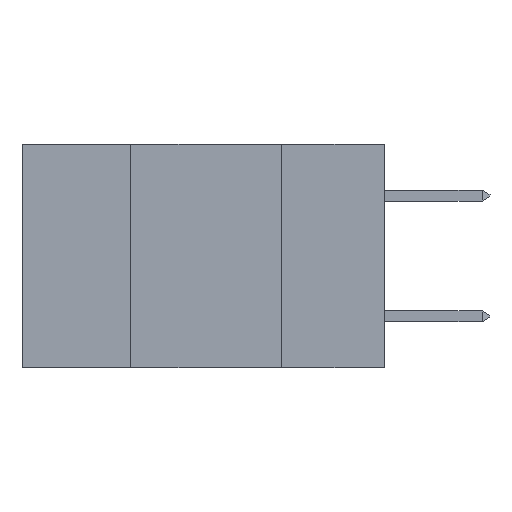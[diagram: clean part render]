
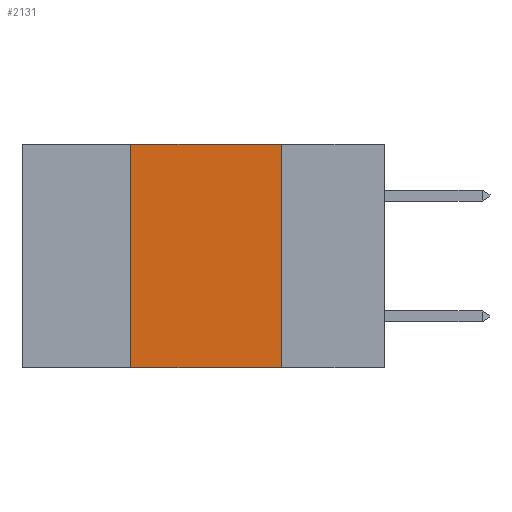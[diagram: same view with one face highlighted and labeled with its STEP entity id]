
A CAD part, left-side view. The second image highlights one B-rep face of the part: STEP entity #2131.
In plain terms, the highlighted planar face has unit normal (-1, 0, 0).
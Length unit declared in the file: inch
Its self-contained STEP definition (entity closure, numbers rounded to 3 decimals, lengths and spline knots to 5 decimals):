
#413 = CARTESIAN_POINT ( 'NONE',  ( 0., 0.42, 0. ) ) ;
#755 = LINE ( 'NONE', #12786, #13240 ) ;
#1171 = CARTESIAN_POINT ( 'NONE',  ( 0., 0.17, -0.37 ) ) ;
#1520 = VERTEX_POINT ( 'NONE', #1171 ) ;
#1821 = VERTEX_POINT ( 'NONE', #7901 ) ;
#2131 = ADVANCED_FACE ( 'NONE', ( #11432 ), #11680, .F. ) ;
#2383 = LINE ( 'NONE', #6045, #12382 ) ;
#2476 = VECTOR ( 'NONE', #11232, 39.37008 ) ;
#2914 = DIRECTION ( 'NONE',  ( 0., 0., 1. ) ) ;
#4854 = LINE ( 'NONE', #413, #14025 ) ;
#5162 = CARTESIAN_POINT ( 'NONE',  ( 0., 0.42, 0. ) ) ;
#6045 = CARTESIAN_POINT ( 'NONE',  ( 0., 0.6, 0. ) ) ;
#6496 = CARTESIAN_POINT ( 'NONE',  ( 0., 0.17, 0. ) ) ;
#6823 = DIRECTION ( 'NONE',  ( 0., -1., 0. ) ) ;
#6924 = DIRECTION ( 'NONE',  ( 1., 0., 0. ) ) ;
#6982 = EDGE_LOOP ( 'NONE', ( #10918, #13888, #10572, #9052 ) ) ;
#7901 = CARTESIAN_POINT ( 'NONE',  ( 0., 0.42, -0.37 ) ) ;
#8477 = EDGE_CURVE ( 'NONE', #1821, #15465, #4854, .T. ) ;
#9052 = ORIENTED_EDGE ( 'NONE', *, *, #14442, .T. ) ;
#10051 = CARTESIAN_POINT ( 'NONE',  ( 0., 0.17, 0. ) ) ;
#10572 = ORIENTED_EDGE ( 'NONE', *, *, #8477, .F. ) ;
#10918 = ORIENTED_EDGE ( 'NONE', *, *, #10987, .F. ) ;
#10987 = EDGE_CURVE ( 'NONE', #14907, #1520, #11728, .T. ) ;
#11232 = DIRECTION ( 'NONE',  ( 0., 0., -1. ) ) ;
#11296 = AXIS2_PLACEMENT_3D ( 'NONE', #12883, #6924, #15204 ) ;
#11432 = FACE_OUTER_BOUND ( 'NONE', #6982, .T. ) ;
#11442 = EDGE_CURVE ( 'NONE', #15465, #14907, #2383, .T. ) ;
#11680 = PLANE ( 'NONE',  #11296 ) ;
#11728 = LINE ( 'NONE', #10051, #2476 ) ;
#12382 = VECTOR ( 'NONE', #14380, 39.37008 ) ;
#12786 = CARTESIAN_POINT ( 'NONE',  ( 0., 0.6, -0.37 ) ) ;
#12883 = CARTESIAN_POINT ( 'NONE',  ( 0., 0.6, 0. ) ) ;
#13240 = VECTOR ( 'NONE', #6823, 39.37008 ) ;
#13888 = ORIENTED_EDGE ( 'NONE', *, *, #11442, .F. ) ;
#14025 = VECTOR ( 'NONE', #2914, 39.37008 ) ;
#14380 = DIRECTION ( 'NONE',  ( 0., -1., 0. ) ) ;
#14442 = EDGE_CURVE ( 'NONE', #1821, #1520, #755, .T. ) ;
#14907 = VERTEX_POINT ( 'NONE', #6496 ) ;
#15204 = DIRECTION ( 'NONE',  ( 0., 0., -1. ) ) ;
#15465 = VERTEX_POINT ( 'NONE', #5162 ) ;
